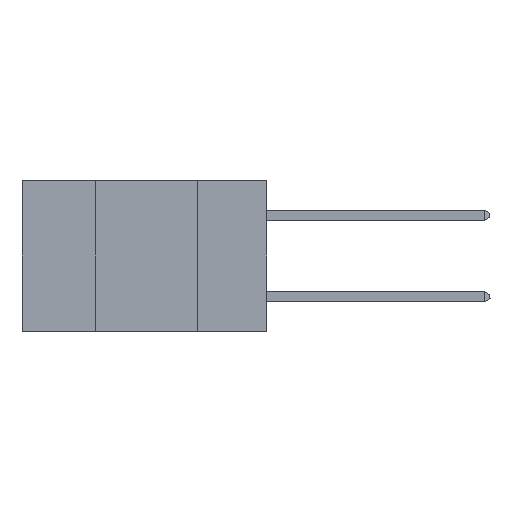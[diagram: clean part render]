
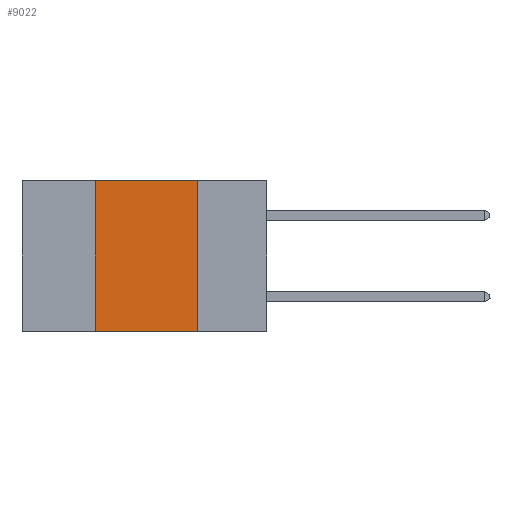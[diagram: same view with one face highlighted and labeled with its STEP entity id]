
A CAD part, left-side view. The second image highlights one B-rep face of the part: STEP entity #9022.
In plain terms, the highlighted planar face has unit normal (-1, 0, 0).
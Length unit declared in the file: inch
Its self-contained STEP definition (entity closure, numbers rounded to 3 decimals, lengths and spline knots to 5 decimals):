
#231 = ORIENTED_EDGE ( 'NONE', *, *, #4239, .T. ) ;
#605 = CARTESIAN_POINT ( 'NONE',  ( 0., 0.17, -0.37 ) ) ;
#649 = CARTESIAN_POINT ( 'NONE',  ( 0., 0.6, 0. ) ) ;
#674 = VERTEX_POINT ( 'NONE', #2675 ) ;
#828 = LINE ( 'NONE', #2668, #2685 ) ;
#1234 = EDGE_CURVE ( 'NONE', #674, #5183, #828, .T. ) ;
#1465 = DIRECTION ( 'NONE',  ( 1., 0., 0. ) ) ;
#1531 = LINE ( 'NONE', #8920, #8613 ) ;
#1954 = LINE ( 'NONE', #2192, #3754 ) ;
#2000 = AXIS2_PLACEMENT_3D ( 'NONE', #649, #1465, #6573 ) ;
#2192 = CARTESIAN_POINT ( 'NONE',  ( 0., 0.6, 0. ) ) ;
#2400 = VERTEX_POINT ( 'NONE', #6695 ) ;
#2668 = CARTESIAN_POINT ( 'NONE',  ( 0., 0.17, 0. ) ) ;
#2675 = CARTESIAN_POINT ( 'NONE',  ( 0., 0.17, 0. ) ) ;
#2685 = VECTOR ( 'NONE', #3147, 39.37008 ) ;
#2973 = ORIENTED_EDGE ( 'NONE', *, *, #1234, .F. ) ;
#3147 = DIRECTION ( 'NONE',  ( 0., 0., -1. ) ) ;
#3271 = ORIENTED_EDGE ( 'NONE', *, *, #6857, .F. ) ;
#3601 = VECTOR ( 'NONE', #6723, 39.37008 ) ;
#3754 = VECTOR ( 'NONE', #3924, 39.37008 ) ;
#3826 = LINE ( 'NONE', #8960, #3601 ) ;
#3924 = DIRECTION ( 'NONE',  ( 0., -1., 0. ) ) ;
#4239 = EDGE_CURVE ( 'NONE', #2400, #5183, #3826, .T. ) ;
#4495 = VERTEX_POINT ( 'NONE', #5399 ) ;
#5183 = VERTEX_POINT ( 'NONE', #605 ) ;
#5191 = DIRECTION ( 'NONE',  ( 0., 0., 1. ) ) ;
#5399 = CARTESIAN_POINT ( 'NONE',  ( 0., 0.42, 0. ) ) ;
#6019 = ORIENTED_EDGE ( 'NONE', *, *, #9019, .F. ) ;
#6573 = DIRECTION ( 'NONE',  ( 0., 0., -1. ) ) ;
#6695 = CARTESIAN_POINT ( 'NONE',  ( 0., 0.42, -0.37 ) ) ;
#6723 = DIRECTION ( 'NONE',  ( 0., -1., 0. ) ) ;
#6857 = EDGE_CURVE ( 'NONE', #4495, #674, #1954, .T. ) ;
#8075 = EDGE_LOOP ( 'NONE', ( #2973, #3271, #6019, #231 ) ) ;
#8613 = VECTOR ( 'NONE', #5191, 39.37008 ) ;
#8810 = FACE_OUTER_BOUND ( 'NONE', #8075, .T. ) ;
#8920 = CARTESIAN_POINT ( 'NONE',  ( 0., 0.42, 0. ) ) ;
#8944 = PLANE ( 'NONE',  #2000 ) ;
#8960 = CARTESIAN_POINT ( 'NONE',  ( 0., 0.6, -0.37 ) ) ;
#9019 = EDGE_CURVE ( 'NONE', #2400, #4495, #1531, .T. ) ;
#9022 = ADVANCED_FACE ( 'NONE', ( #8810 ), #8944, .F. ) ;
